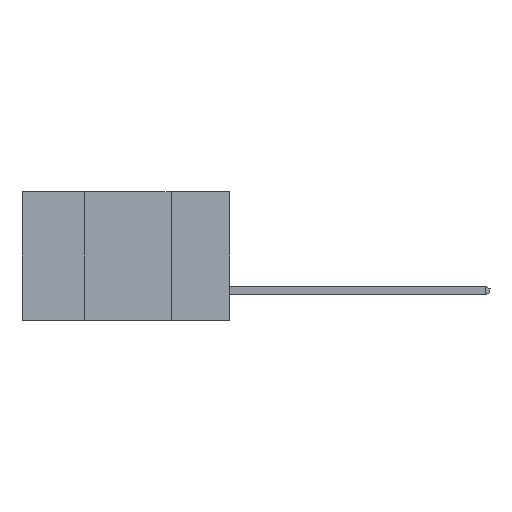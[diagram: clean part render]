
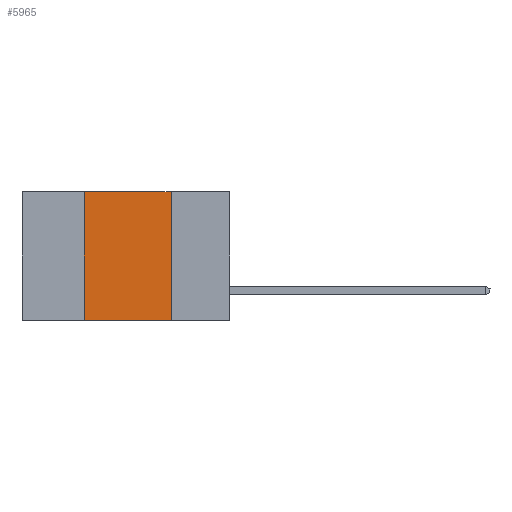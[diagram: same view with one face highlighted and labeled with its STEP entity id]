
A CAD part, left-side view. The second image highlights one B-rep face of the part: STEP entity #5965.
In plain terms, the highlighted planar face has unit normal (-1, 0, 0).
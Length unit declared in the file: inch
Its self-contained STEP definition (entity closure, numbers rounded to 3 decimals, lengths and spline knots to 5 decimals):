
#616 = CARTESIAN_POINT ( 'NONE',  ( 0., 0.6, 0. ) ) ;
#621 = DIRECTION ( 'NONE',  ( 0., 0., 1. ) ) ;
#987 = VERTEX_POINT ( 'NONE', #4694 ) ;
#1097 = LINE ( 'NONE', #7361, #2437 ) ;
#1669 = VERTEX_POINT ( 'NONE', #2088 ) ;
#2088 = CARTESIAN_POINT ( 'NONE',  ( 0., 0.17, -0.37 ) ) ;
#2151 = LINE ( 'NONE', #616, #7790 ) ;
#2437 = VECTOR ( 'NONE', #5930, 39.37008 ) ;
#3096 = DIRECTION ( 'NONE',  ( 0., 0., -1. ) ) ;
#3611 = LINE ( 'NONE', #4528, #5410 ) ;
#3624 = VECTOR ( 'NONE', #7991, 39.37008 ) ;
#3673 = VERTEX_POINT ( 'NONE', #8751 ) ;
#3824 = PLANE ( 'NONE',  #9342 ) ;
#4528 = CARTESIAN_POINT ( 'NONE',  ( 0., 0.42, -0.37 ) ) ;
#4576 = ORIENTED_EDGE ( 'NONE', *, *, #5077, .F. ) ;
#4595 = ORIENTED_EDGE ( 'NONE', *, *, #6848, .F. ) ;
#4694 = CARTESIAN_POINT ( 'NONE',  ( 0., 0.42, 0. ) ) ;
#5077 = EDGE_CURVE ( 'NONE', #987, #9693, #2151, .T. ) ;
#5234 = CARTESIAN_POINT ( 'NONE',  ( 0., 0.17, 0. ) ) ;
#5410 = VECTOR ( 'NONE', #621, 39.37008 ) ;
#5754 = EDGE_CURVE ( 'NONE', #3673, #1669, #1097, .T. ) ;
#5809 = EDGE_LOOP ( 'NONE', ( #9427, #4576, #4595, #5851 ) ) ;
#5851 = ORIENTED_EDGE ( 'NONE', *, *, #5754, .T. ) ;
#5930 = DIRECTION ( 'NONE',  ( 0., -1., 0. ) ) ;
#5965 = ADVANCED_FACE ( 'NONE', ( #7776 ), #3824, .F. ) ;
#6674 = CARTESIAN_POINT ( 'NONE',  ( 0., 0.17, -0.37 ) ) ;
#6848 = EDGE_CURVE ( 'NONE', #3673, #987, #3611, .T. ) ;
#6994 = DIRECTION ( 'NONE',  ( 1., 0., 0. ) ) ;
#7361 = CARTESIAN_POINT ( 'NONE',  ( 0., 0.6, -0.37 ) ) ;
#7776 = FACE_OUTER_BOUND ( 'NONE', #5809, .T. ) ;
#7790 = VECTOR ( 'NONE', #8329, 39.37008 ) ;
#7991 = DIRECTION ( 'NONE',  ( 0., 0., -1. ) ) ;
#8326 = LINE ( 'NONE', #6674, #3624 ) ;
#8329 = DIRECTION ( 'NONE',  ( 0., -1., 0. ) ) ;
#8751 = CARTESIAN_POINT ( 'NONE',  ( 0., 0.42, -0.37 ) ) ;
#9342 = AXIS2_PLACEMENT_3D ( 'NONE', #10090, #6994, #3096 ) ;
#9427 = ORIENTED_EDGE ( 'NONE', *, *, #9588, .F. ) ;
#9588 = EDGE_CURVE ( 'NONE', #9693, #1669, #8326, .T. ) ;
#9693 = VERTEX_POINT ( 'NONE', #5234 ) ;
#10090 = CARTESIAN_POINT ( 'NONE',  ( 0., 0.6, 0. ) ) ;
